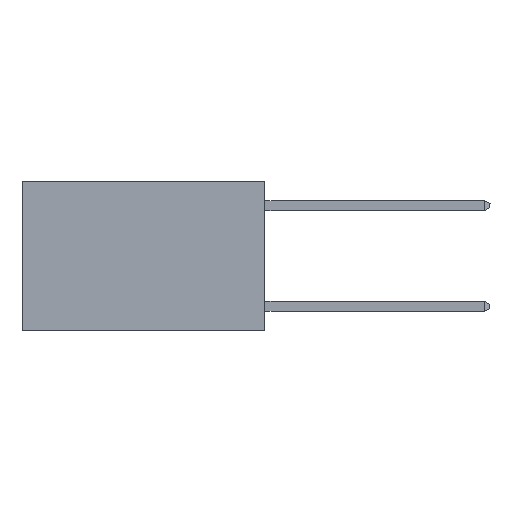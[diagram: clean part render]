
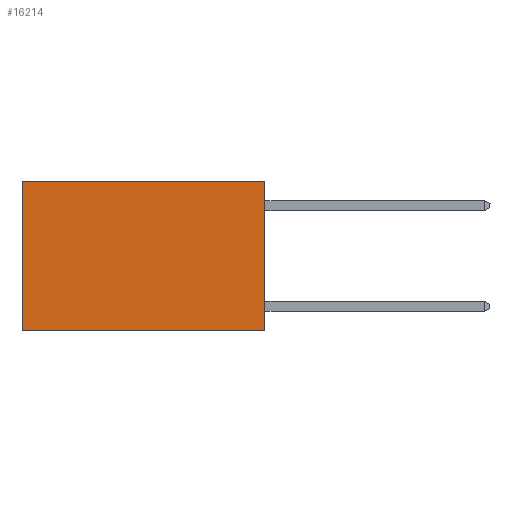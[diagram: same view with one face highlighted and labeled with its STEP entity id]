
A CAD part, left-side view. The second image highlights one B-rep face of the part: STEP entity #16214.
In plain terms, the highlighted planar face has unit normal (-1, 0, 0).
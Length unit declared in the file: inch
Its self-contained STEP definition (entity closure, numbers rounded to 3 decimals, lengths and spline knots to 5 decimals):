
#116 = VECTOR ( 'NONE', #10377, 39.37008 ) ;
#665 = EDGE_LOOP ( 'NONE', ( #7008, #17500, #4436, #22554 ) ) ;
#804 = CARTESIAN_POINT ( 'NONE',  ( 0.2625, 0., 0. ) ) ;
#1366 = VECTOR ( 'NONE', #21669, 39.37008 ) ;
#1618 = VECTOR ( 'NONE', #2563, 39.37008 ) ;
#2559 = FACE_OUTER_BOUND ( 'NONE', #665, .T. ) ;
#2563 = DIRECTION ( 'NONE',  ( 0., 1., 0. ) ) ;
#3301 = CARTESIAN_POINT ( 'NONE',  ( 0.2625, 0., 0. ) ) ;
#4436 = ORIENTED_EDGE ( 'NONE', *, *, #4826, .F. ) ;
#4746 = LINE ( 'NONE', #7002, #9964 ) ;
#4826 = EDGE_CURVE ( 'NONE', #13092, #14154, #30249, .T. ) ;
#6064 = EDGE_CURVE ( 'NONE', #25788, #19865, #30763, .T. ) ;
#7002 = CARTESIAN_POINT ( 'NONE',  ( 0.2625, 0., -0.37 ) ) ;
#7008 = ORIENTED_EDGE ( 'NONE', *, *, #6064, .T. ) ;
#8139 = CARTESIAN_POINT ( 'NONE',  ( 0.2625, 0.6, 0. ) ) ;
#8331 = CARTESIAN_POINT ( 'NONE',  ( 0.2625, 0.6, -0.37 ) ) ;
#8767 = EDGE_CURVE ( 'NONE', #13092, #25788, #9790, .T. ) ;
#8984 = AXIS2_PLACEMENT_3D ( 'NONE', #3301, #10460, #12866 ) ;
#9790 = LINE ( 'NONE', #25989, #1618 ) ;
#9964 = VECTOR ( 'NONE', #23545, 39.37008 ) ;
#10377 = DIRECTION ( 'NONE',  ( 0., 0., -1. ) ) ;
#10460 = DIRECTION ( 'NONE',  ( 1., 0., 0. ) ) ;
#12866 = DIRECTION ( 'NONE',  ( 0., 0., -1. ) ) ;
#13092 = VERTEX_POINT ( 'NONE', #804 ) ;
#14154 = VERTEX_POINT ( 'NONE', #21264 ) ;
#14673 = CARTESIAN_POINT ( 'NONE',  ( 0.2625, 0., 0. ) ) ;
#16214 = ADVANCED_FACE ( 'NONE', ( #2559 ), #17511, .F. ) ;
#17500 = ORIENTED_EDGE ( 'NONE', *, *, #30413, .F. ) ;
#17511 = PLANE ( 'NONE',  #8984 ) ;
#19710 = CARTESIAN_POINT ( 'NONE',  ( 0.2625, 0.6, 0. ) ) ;
#19865 = VERTEX_POINT ( 'NONE', #8331 ) ;
#21264 = CARTESIAN_POINT ( 'NONE',  ( 0.2625, 0., -0.37 ) ) ;
#21669 = DIRECTION ( 'NONE',  ( 0., 0., -1. ) ) ;
#22554 = ORIENTED_EDGE ( 'NONE', *, *, #8767, .T. ) ;
#23545 = DIRECTION ( 'NONE',  ( 0., 1., 0. ) ) ;
#25788 = VERTEX_POINT ( 'NONE', #8139 ) ;
#25989 = CARTESIAN_POINT ( 'NONE',  ( 0.2625, 0., 0. ) ) ;
#30249 = LINE ( 'NONE', #14673, #116 ) ;
#30413 = EDGE_CURVE ( 'NONE', #14154, #19865, #4746, .T. ) ;
#30763 = LINE ( 'NONE', #19710, #1366 ) ;
